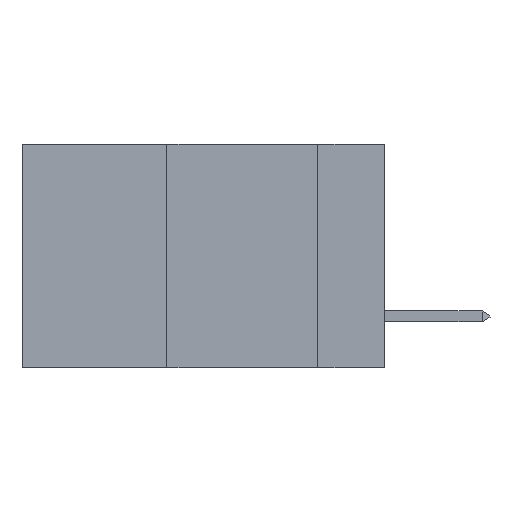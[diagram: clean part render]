
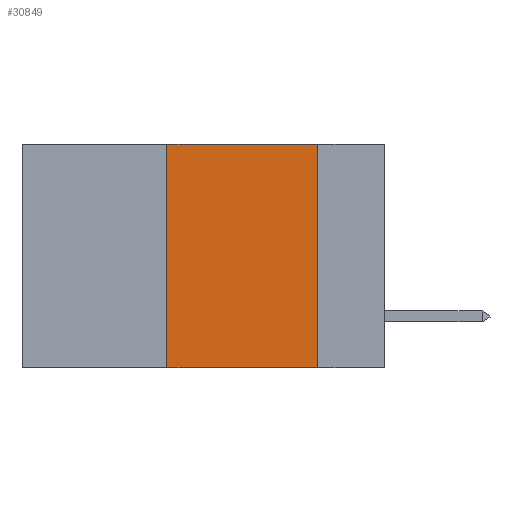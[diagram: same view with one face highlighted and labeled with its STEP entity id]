
A CAD part, left-side view. The second image highlights one B-rep face of the part: STEP entity #30849.
In plain terms, the highlighted planar face has unit normal (-1, 0, 0).
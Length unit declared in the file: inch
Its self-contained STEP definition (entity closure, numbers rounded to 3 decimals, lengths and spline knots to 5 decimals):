
#1925 = FACE_OUTER_BOUND ( 'NONE', #4370, .T. ) ;
#2558 = DIRECTION ( 'NONE',  ( 0., -1., 0. ) ) ;
#4370 = EDGE_LOOP ( 'NONE', ( #22028, #22620, #35726, #22150 ) ) ;
#4921 = DIRECTION ( 'NONE',  ( 0., 0., -1. ) ) ;
#7542 = CARTESIAN_POINT ( 'NONE',  ( 0., 0.11, 0. ) ) ;
#7872 = DIRECTION ( 'NONE',  ( 0., -1., 0. ) ) ;
#8475 = EDGE_CURVE ( 'NONE', #27779, #37071, #30009, .T. ) ;
#9142 = LINE ( 'NONE', #39942, #17856 ) ;
#9869 = EDGE_CURVE ( 'NONE', #37071, #31497, #23054, .T. ) ;
#10366 = PLANE ( 'NONE',  #11473 ) ;
#11473 = AXIS2_PLACEMENT_3D ( 'NONE', #32862, #13645, #36104 ) ;
#13496 = VECTOR ( 'NONE', #2558, 39.37008 ) ;
#13645 = DIRECTION ( 'NONE',  ( 1., 0., 0. ) ) ;
#15139 = CARTESIAN_POINT ( 'NONE',  ( 0., 0.11, -0.37 ) ) ;
#17827 = EDGE_CURVE ( 'NONE', #31497, #33649, #19687, .T. ) ;
#17856 = VECTOR ( 'NONE', #7872, 39.37008 ) ;
#19122 = CARTESIAN_POINT ( 'NONE',  ( 0., 0.36, 0. ) ) ;
#19598 = CARTESIAN_POINT ( 'NONE',  ( 0., 0.36, 0. ) ) ;
#19687 = LINE ( 'NONE', #40250, #35719 ) ;
#22028 = ORIENTED_EDGE ( 'NONE', *, *, #17827, .F. ) ;
#22150 = ORIENTED_EDGE ( 'NONE', *, *, #32814, .T. ) ;
#22620 = ORIENTED_EDGE ( 'NONE', *, *, #9869, .F. ) ;
#23054 = LINE ( 'NONE', #24421, #13496 ) ;
#24421 = CARTESIAN_POINT ( 'NONE',  ( 0., 0.6, 0. ) ) ;
#27779 = VERTEX_POINT ( 'NONE', #41586 ) ;
#27893 = DIRECTION ( 'NONE',  ( 0., 0., 1. ) ) ;
#30009 = LINE ( 'NONE', #19598, #37517 ) ;
#30849 = ADVANCED_FACE ( 'NONE', ( #1925 ), #10366, .F. ) ;
#31497 = VERTEX_POINT ( 'NONE', #7542 ) ;
#32814 = EDGE_CURVE ( 'NONE', #27779, #33649, #9142, .T. ) ;
#32862 = CARTESIAN_POINT ( 'NONE',  ( 0., 0.6, 0. ) ) ;
#33649 = VERTEX_POINT ( 'NONE', #15139 ) ;
#35719 = VECTOR ( 'NONE', #4921, 39.37008 ) ;
#35726 = ORIENTED_EDGE ( 'NONE', *, *, #8475, .F. ) ;
#36104 = DIRECTION ( 'NONE',  ( 0., 0., -1. ) ) ;
#37071 = VERTEX_POINT ( 'NONE', #19122 ) ;
#37517 = VECTOR ( 'NONE', #27893, 39.37008 ) ;
#39942 = CARTESIAN_POINT ( 'NONE',  ( 0., 0.6, -0.37 ) ) ;
#40250 = CARTESIAN_POINT ( 'NONE',  ( 0., 0.11, 0. ) ) ;
#41586 = CARTESIAN_POINT ( 'NONE',  ( 0., 0.36, -0.37 ) ) ;
